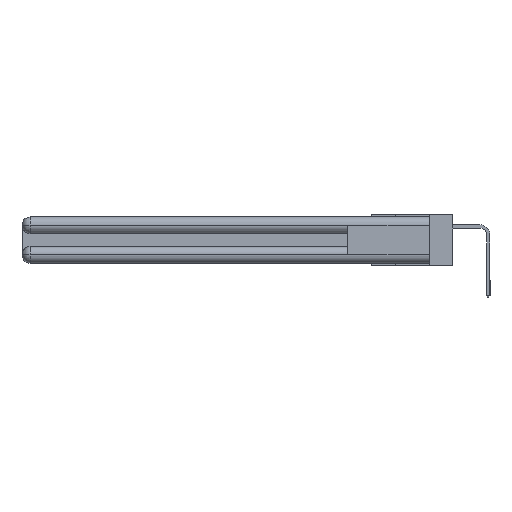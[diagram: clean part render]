
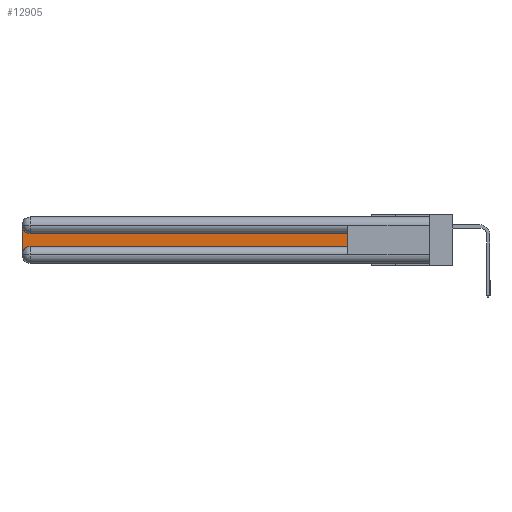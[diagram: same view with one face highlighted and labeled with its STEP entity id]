
A CAD part, left-side view. The second image highlights one B-rep face of the part: STEP entity #12905.
In plain terms, the highlighted planar face has unit normal (-1, 0, 0).
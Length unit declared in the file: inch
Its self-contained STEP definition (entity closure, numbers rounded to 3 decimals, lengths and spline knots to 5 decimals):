
#689 = CARTESIAN_POINT ( 'NONE',  ( 0.075, 3., -0.1225 ) ) ;
#3891 = LINE ( 'NONE', #18473, #13009 ) ;
#4397 = ORIENTED_EDGE ( 'NONE', *, *, #15931, .T. ) ;
#4574 = CARTESIAN_POINT ( 'NONE',  ( 0.075, 2.94, -0.2175 ) ) ;
#4630 = ORIENTED_EDGE ( 'NONE', *, *, #27195, .T. ) ;
#4936 = LINE ( 'NONE', #31603, #10472 ) ;
#6505 = DIRECTION ( 'NONE',  ( 0., 0., -1. ) ) ;
#6516 = CARTESIAN_POINT ( 'NONE',  ( 0.075, 2.94, -0.0625 ) ) ;
#6871 = VERTEX_POINT ( 'NONE', #4574 ) ;
#7600 = VERTEX_POINT ( 'NONE', #10418 ) ;
#7834 = EDGE_CURVE ( 'NONE', #13562, #15965, #3891, .T. ) ;
#8524 = PLANE ( 'NONE',  #26180 ) ;
#8649 = EDGE_LOOP ( 'NONE', ( #20292, #18702, #16411, #4630, #4397, #22669 ) ) ;
#8937 = LINE ( 'NONE', #30030, #18412 ) ;
#9003 = CARTESIAN_POINT ( 'NONE',  ( 0.075, 0.6, -0.1225 ) ) ;
#9005 = DIRECTION ( 'NONE',  ( 0., 0., -1. ) ) ;
#9204 = DIRECTION ( 'NONE',  ( 0., 1., 0. ) ) ;
#9309 = DIRECTION ( 'NONE',  ( 1., 0., 0. ) ) ;
#9741 = CARTESIAN_POINT ( 'NONE',  ( 0.075, 3., -0.0625 ) ) ;
#10418 = CARTESIAN_POINT ( 'NONE',  ( 0.075, 2.94, -0.1225 ) ) ;
#10472 = VECTOR ( 'NONE', #6505, 39.37008 ) ;
#10524 = CARTESIAN_POINT ( 'NONE',  ( 0.075, 3., -0.2775 ) ) ;
#10949 = DIRECTION ( 'NONE',  ( 1., 0., 0. ) ) ;
#10963 = DIRECTION ( 'NONE',  ( 0., 0., 1. ) ) ;
#11854 = DIRECTION ( 'NONE',  ( 0., 0., -1. ) ) ;
#12267 = FACE_OUTER_BOUND ( 'NONE', #8649, .T. ) ;
#12905 = ADVANCED_FACE ( 'NONE', ( #12267 ), #8524, .F. ) ;
#13009 = VECTOR ( 'NONE', #10963, 39.37008 ) ;
#13488 = LINE ( 'NONE', #9003, #18214 ) ;
#13559 = VERTEX_POINT ( 'NONE', #9741 ) ;
#13562 = VERTEX_POINT ( 'NONE', #19582 ) ;
#15003 = EDGE_CURVE ( 'NONE', #7600, #13559, #28787, .T. ) ;
#15169 = DIRECTION ( 'NONE',  ( 0., -1., 0. ) ) ;
#15931 = EDGE_CURVE ( 'NONE', #6871, #13562, #8937, .T. ) ;
#15965 = VERTEX_POINT ( 'NONE', #25126 ) ;
#16411 = ORIENTED_EDGE ( 'NONE', *, *, #18169, .T. ) ;
#18169 = EDGE_CURVE ( 'NONE', #13559, #18440, #4936, .T. ) ;
#18214 = VECTOR ( 'NONE', #9204, 39.37008 ) ;
#18412 = VECTOR ( 'NONE', #15169, 39.37008 ) ;
#18440 = VERTEX_POINT ( 'NONE', #10524 ) ;
#18473 = CARTESIAN_POINT ( 'NONE',  ( 0.075, 0.6, -0.2175 ) ) ;
#18702 = ORIENTED_EDGE ( 'NONE', *, *, #15003, .T. ) ;
#19484 = CARTESIAN_POINT ( 'NONE',  ( 0.075, 2.94, -0.2775 ) ) ;
#19582 = CARTESIAN_POINT ( 'NONE',  ( 0.075, 0.6, -0.2175 ) ) ;
#20292 = ORIENTED_EDGE ( 'NONE', *, *, #20407, .T. ) ;
#20407 = EDGE_CURVE ( 'NONE', #15965, #7600, #13488, .T. ) ;
#22669 = ORIENTED_EDGE ( 'NONE', *, *, #7834, .T. ) ;
#22947 = CIRCLE ( 'NONE', #25610, 0.06 ) ;
#23661 = DIRECTION ( 'NONE',  ( 0., 0., -1. ) ) ;
#25126 = CARTESIAN_POINT ( 'NONE',  ( 0.075, 0.6, -0.1225 ) ) ;
#25610 = AXIS2_PLACEMENT_3D ( 'NONE', #19484, #32177, #9005 ) ;
#26180 = AXIS2_PLACEMENT_3D ( 'NONE', #689, #10949, #23661 ) ;
#27195 = EDGE_CURVE ( 'NONE', #18440, #6871, #22947, .T. ) ;
#28594 = AXIS2_PLACEMENT_3D ( 'NONE', #6516, #9309, #11854 ) ;
#28787 = CIRCLE ( 'NONE', #28594, 0.06 ) ;
#30030 = CARTESIAN_POINT ( 'NONE',  ( 0.075, 0.6, -0.2175 ) ) ;
#31603 = CARTESIAN_POINT ( 'NONE',  ( 0.075, 3., -0.2175 ) ) ;
#32177 = DIRECTION ( 'NONE',  ( 1., 0., 0. ) ) ;
